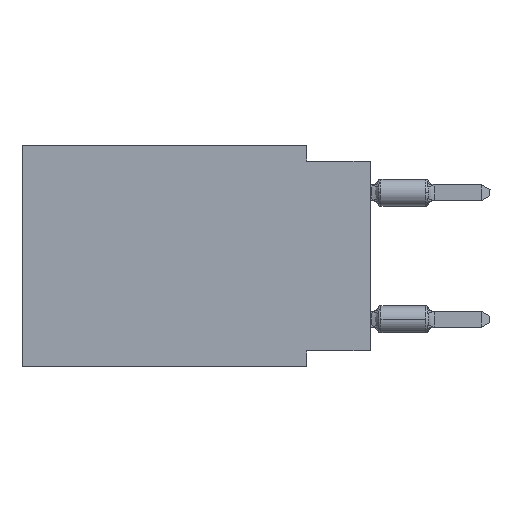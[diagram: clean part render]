
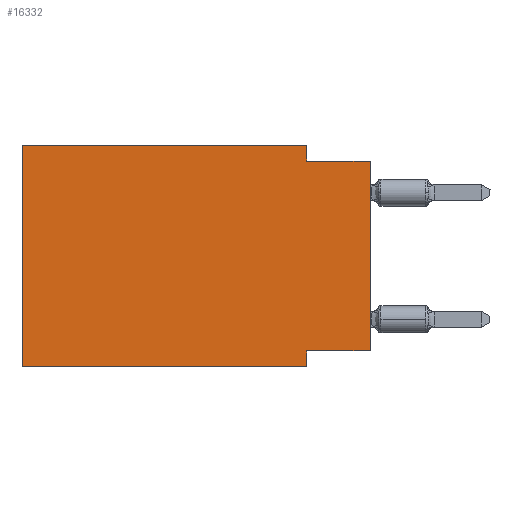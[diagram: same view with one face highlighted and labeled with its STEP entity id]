
A CAD part, left-side view. The second image highlights one B-rep face of the part: STEP entity #16332.
In plain terms, the highlighted planar face has unit normal (-1, 0, 0).
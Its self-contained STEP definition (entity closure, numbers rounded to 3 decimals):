
#1130 = VECTOR ( 'NONE', #52058, 1000. ) ;
#1135 = CARTESIAN_POINT ( 'NONE',  ( 0., 13.97, 0. ) ) ;
#1158 = LINE ( 'NONE', #35091, #1130 ) ;
#1488 = CARTESIAN_POINT ( 'NONE',  ( 0., 13.97, -8.89 ) ) ;
#1976 = ORIENTED_EDGE ( 'NONE', *, *, #52797, .F. ) ;
#3846 = CARTESIAN_POINT ( 'NONE',  ( 0., 2.54, -8.89 ) ) ;
#4254 = VECTOR ( 'NONE', #53321, 1000. ) ;
#4603 = DIRECTION ( 'NONE',  ( 0., 0., -1. ) ) ;
#4721 = DIRECTION ( 'NONE',  ( 0., 0., -1. ) ) ;
#5013 = VERTEX_POINT ( 'NONE', #48072 ) ;
#5036 = FACE_OUTER_BOUND ( 'NONE', #26951, .T. ) ;
#5075 = LINE ( 'NONE', #51795, #54803 ) ;
#5369 = CARTESIAN_POINT ( 'NONE',  ( 0., 13.97, 0. ) ) ;
#5430 = LINE ( 'NONE', #42725, #25696 ) ;
#6714 = VECTOR ( 'NONE', #26222, 1000. ) ;
#9052 = EDGE_CURVE ( 'NONE', #39259, #20418, #20220, .T. ) ;
#9243 = CARTESIAN_POINT ( 'NONE',  ( 0., 13.97, 0. ) ) ;
#10743 = ORIENTED_EDGE ( 'NONE', *, *, #9052, .F. ) ;
#11597 = CARTESIAN_POINT ( 'NONE',  ( 0., 13.97, 0. ) ) ;
#13512 = DIRECTION ( 'NONE',  ( 0., 1., 0. ) ) ;
#13699 = ORIENTED_EDGE ( 'NONE', *, *, #28161, .F. ) ;
#16332 = ADVANCED_FACE ( 'NONE', ( #5036 ), #26463, .F. ) ;
#17412 = CARTESIAN_POINT ( 'NONE',  ( 0., 0., -0.635 ) ) ;
#17653 = LINE ( 'NONE', #1488, #18146 ) ;
#18146 = VECTOR ( 'NONE', #43787, 1000. ) ;
#18234 = LINE ( 'NONE', #39377, #29135 ) ;
#18694 = CARTESIAN_POINT ( 'NONE',  ( 0., 0., -8.255 ) ) ;
#18922 = DIRECTION ( 'NONE',  ( 0., 0., -1. ) ) ;
#19801 = VERTEX_POINT ( 'NONE', #17412 ) ;
#20220 = LINE ( 'NONE', #11597, #4254 ) ;
#20418 = VERTEX_POINT ( 'NONE', #5369 ) ;
#21765 = EDGE_CURVE ( 'NONE', #25056, #5013, #18234, .T. ) ;
#25056 = VERTEX_POINT ( 'NONE', #18694 ) ;
#25696 = VECTOR ( 'NONE', #4603, 1000. ) ;
#25864 = VERTEX_POINT ( 'NONE', #3846 ) ;
#26222 = DIRECTION ( 'NONE',  ( 0., -1., 0. ) ) ;
#26223 = VECTOR ( 'NONE', #4721, 1000. ) ;
#26463 = PLANE ( 'NONE',  #27818 ) ;
#26951 = EDGE_LOOP ( 'NONE', ( #37276, #13699, #1976, #47265, #10743, #38534, #45932, #34316 ) ) ;
#27818 = AXIS2_PLACEMENT_3D ( 'NONE', #1135, #48134, #18922 ) ;
#28161 = EDGE_CURVE ( 'NONE', #34392, #19801, #1158, .T. ) ;
#29135 = VECTOR ( 'NONE', #13512, 1000. ) ;
#29578 = DIRECTION ( 'NONE',  ( 0., 0., 1. ) ) ;
#34274 = EDGE_CURVE ( 'NONE', #25056, #19801, #5075, .T. ) ;
#34316 = ORIENTED_EDGE ( 'NONE', *, *, #21765, .F. ) ;
#34392 = VERTEX_POINT ( 'NONE', #40111 ) ;
#35091 = CARTESIAN_POINT ( 'NONE',  ( 0., 0., -0.635 ) ) ;
#37276 = ORIENTED_EDGE ( 'NONE', *, *, #34274, .T. ) ;
#38534 = ORIENTED_EDGE ( 'NONE', *, *, #50039, .T. ) ;
#38662 = EDGE_CURVE ( 'NONE', #5013, #25864, #5430, .T. ) ;
#39259 = VERTEX_POINT ( 'NONE', #44845 ) ;
#39377 = CARTESIAN_POINT ( 'NONE',  ( 0., 0., -8.255 ) ) ;
#40111 = CARTESIAN_POINT ( 'NONE',  ( 0., 2.54, -0.635 ) ) ;
#42281 = LINE ( 'NONE', #42837, #26223 ) ;
#42725 = CARTESIAN_POINT ( 'NONE',  ( 0., 2.54, -8.89 ) ) ;
#42837 = CARTESIAN_POINT ( 'NONE',  ( 0., 2.54, 0. ) ) ;
#43787 = DIRECTION ( 'NONE',  ( 0., -1., 0. ) ) ;
#44845 = CARTESIAN_POINT ( 'NONE',  ( 0., 13.97, -8.89 ) ) ;
#44959 = VERTEX_POINT ( 'NONE', #52908 ) ;
#45932 = ORIENTED_EDGE ( 'NONE', *, *, #38662, .F. ) ;
#47091 = LINE ( 'NONE', #9243, #6714 ) ;
#47265 = ORIENTED_EDGE ( 'NONE', *, *, #53633, .F. ) ;
#48072 = CARTESIAN_POINT ( 'NONE',  ( 0., 2.54, -8.255 ) ) ;
#48134 = DIRECTION ( 'NONE',  ( 1., 0., 0. ) ) ;
#50039 = EDGE_CURVE ( 'NONE', #39259, #25864, #17653, .T. ) ;
#51795 = CARTESIAN_POINT ( 'NONE',  ( 0., 0., 0. ) ) ;
#52058 = DIRECTION ( 'NONE',  ( 0., -1., 0. ) ) ;
#52797 = EDGE_CURVE ( 'NONE', #44959, #34392, #42281, .T. ) ;
#52908 = CARTESIAN_POINT ( 'NONE',  ( 0., 2.54, 0. ) ) ;
#53321 = DIRECTION ( 'NONE',  ( 0., 0., 1. ) ) ;
#53633 = EDGE_CURVE ( 'NONE', #20418, #44959, #47091, .T. ) ;
#54803 = VECTOR ( 'NONE', #29578, 1000. ) ;
